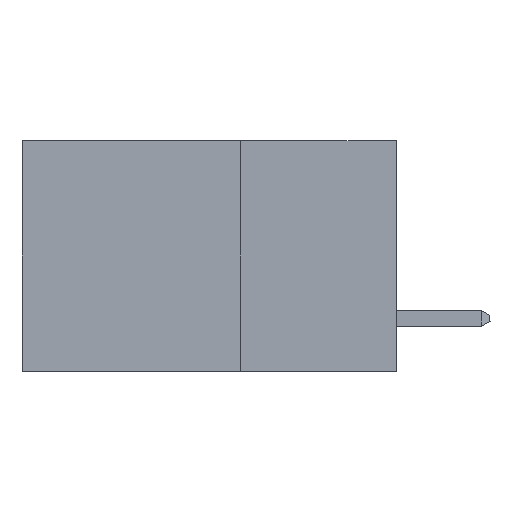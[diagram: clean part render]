
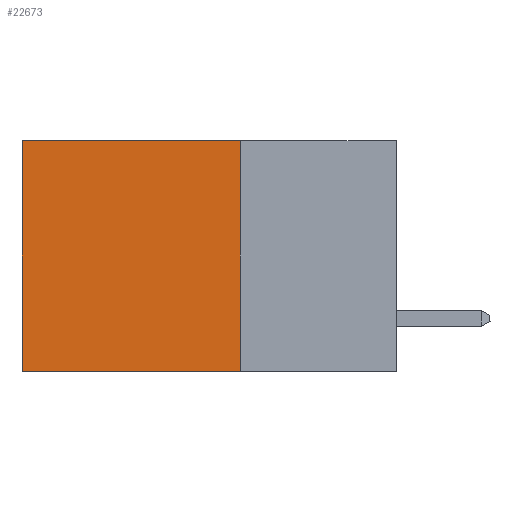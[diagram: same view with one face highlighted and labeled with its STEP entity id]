
A CAD part, left-side view. The second image highlights one B-rep face of the part: STEP entity #22673.
In plain terms, the highlighted planar face has unit normal (-1, 0, 0).
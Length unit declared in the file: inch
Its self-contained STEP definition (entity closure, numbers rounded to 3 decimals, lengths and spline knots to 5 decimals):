
#451 = PLANE ( 'NONE',  #25729 ) ;
#553 = DIRECTION ( 'NONE',  ( 1., 0., 0. ) ) ;
#719 = CARTESIAN_POINT ( 'NONE',  ( 0.298, 0.25, 0. ) ) ;
#956 = LINE ( 'NONE', #14490, #7172 ) ;
#2004 = DIRECTION ( 'NONE',  ( 0., 1., 0. ) ) ;
#2681 = ORIENTED_EDGE ( 'NONE', *, *, #26141, .T. ) ;
#3658 = LINE ( 'NONE', #10529, #25063 ) ;
#4134 = LINE ( 'NONE', #21829, #9673 ) ;
#5092 = CARTESIAN_POINT ( 'NONE',  ( 0.298, 0.25, -0.37 ) ) ;
#5241 = ORIENTED_EDGE ( 'NONE', *, *, #5844, .F. ) ;
#5844 = EDGE_CURVE ( 'NONE', #12069, #19413, #16719, .T. ) ;
#7172 = VECTOR ( 'NONE', #2004, 39.37008 ) ;
#8138 = EDGE_LOOP ( 'NONE', ( #9535, #24099, #5241, #2681 ) ) ;
#9385 = DIRECTION ( 'NONE',  ( 0., 1., 0. ) ) ;
#9535 = ORIENTED_EDGE ( 'NONE', *, *, #23920, .T. ) ;
#9673 = VECTOR ( 'NONE', #9385, 39.37008 ) ;
#10529 = CARTESIAN_POINT ( 'NONE',  ( 0.298, 0.6, 0. ) ) ;
#11175 = VECTOR ( 'NONE', #20381, 39.37008 ) ;
#12069 = VERTEX_POINT ( 'NONE', #719 ) ;
#13075 = CARTESIAN_POINT ( 'NONE',  ( 0.298, 0.25, 0. ) ) ;
#14490 = CARTESIAN_POINT ( 'NONE',  ( 0.298, 0.25, -0.37 ) ) ;
#15168 = DIRECTION ( 'NONE',  ( 0., 0., -1. ) ) ;
#16719 = LINE ( 'NONE', #18297, #11175 ) ;
#16833 = DIRECTION ( 'NONE',  ( 0., 0., -1. ) ) ;
#17512 = CARTESIAN_POINT ( 'NONE',  ( 0.298, 0.6, -0.37 ) ) ;
#18297 = CARTESIAN_POINT ( 'NONE',  ( 0.298, 0.25, 0. ) ) ;
#19413 = VERTEX_POINT ( 'NONE', #5092 ) ;
#20339 = FACE_OUTER_BOUND ( 'NONE', #8138, .T. ) ;
#20381 = DIRECTION ( 'NONE',  ( 0., 0., -1. ) ) ;
#20534 = VERTEX_POINT ( 'NONE', #17512 ) ;
#20680 = VERTEX_POINT ( 'NONE', #24154 ) ;
#20871 = EDGE_CURVE ( 'NONE', #19413, #20534, #956, .T. ) ;
#21829 = CARTESIAN_POINT ( 'NONE',  ( 0.298, 0.25, 0. ) ) ;
#22673 = ADVANCED_FACE ( 'NONE', ( #20339 ), #451, .F. ) ;
#23920 = EDGE_CURVE ( 'NONE', #20680, #20534, #3658, .T. ) ;
#24099 = ORIENTED_EDGE ( 'NONE', *, *, #20871, .F. ) ;
#24154 = CARTESIAN_POINT ( 'NONE',  ( 0.298, 0.6, 0. ) ) ;
#25063 = VECTOR ( 'NONE', #16833, 39.37008 ) ;
#25729 = AXIS2_PLACEMENT_3D ( 'NONE', #13075, #553, #15168 ) ;
#26141 = EDGE_CURVE ( 'NONE', #12069, #20680, #4134, .T. ) ;
